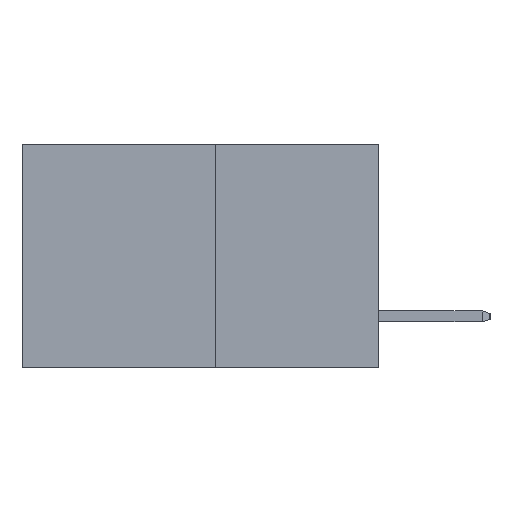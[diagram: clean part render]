
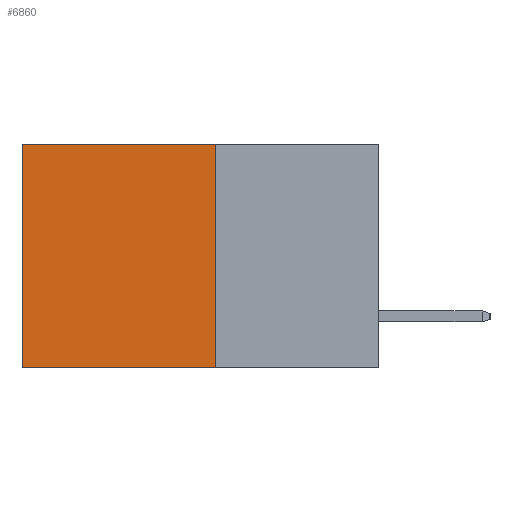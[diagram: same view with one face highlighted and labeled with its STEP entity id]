
A CAD part, left-side view. The second image highlights one B-rep face of the part: STEP entity #6860.
In plain terms, the highlighted planar face has unit normal (-1, 0, 0).
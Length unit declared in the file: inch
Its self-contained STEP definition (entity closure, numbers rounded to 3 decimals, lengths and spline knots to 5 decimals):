
#14 = PLANE ( 'NONE',  #4374 ) ;
#147 = LINE ( 'NONE', #5275, #4679 ) ;
#233 = LINE ( 'NONE', #394, #4769 ) ;
#394 = CARTESIAN_POINT ( 'NONE',  ( 0.277, 0.27, -0.37 ) ) ;
#927 = EDGE_CURVE ( 'NONE', #1650, #7988, #4878, .T. ) ;
#1343 = EDGE_CURVE ( 'NONE', #1881, #6970, #4865, .T. ) ;
#1384 = ORIENTED_EDGE ( 'NONE', *, *, #1343, .T. ) ;
#1650 = VERTEX_POINT ( 'NONE', #10716 ) ;
#1881 = VERTEX_POINT ( 'NONE', #8391 ) ;
#1893 = DIRECTION ( 'NONE',  ( 1., 0., 0. ) ) ;
#2575 = CARTESIAN_POINT ( 'NONE',  ( 0.277, 0.27, -0.37 ) ) ;
#3028 = FACE_OUTER_BOUND ( 'NONE', #7648, .T. ) ;
#3999 = ORIENTED_EDGE ( 'NONE', *, *, #5918, .F. ) ;
#4323 = VECTOR ( 'NONE', #5070, 39.37008 ) ;
#4374 = AXIS2_PLACEMENT_3D ( 'NONE', #7253, #1893, #8123 ) ;
#4579 = VECTOR ( 'NONE', #7801, 39.37008 ) ;
#4679 = VECTOR ( 'NONE', #6206, 39.37008 ) ;
#4769 = VECTOR ( 'NONE', #6738, 39.37008 ) ;
#4865 = LINE ( 'NONE', #9059, #4579 ) ;
#4878 = LINE ( 'NONE', #2575, #4323 ) ;
#5070 = DIRECTION ( 'NONE',  ( 0., 0., -1. ) ) ;
#5275 = CARTESIAN_POINT ( 'NONE',  ( 0.277, 0.27, 0. ) ) ;
#5918 = EDGE_CURVE ( 'NONE', #7988, #6970, #233, .T. ) ;
#6206 = DIRECTION ( 'NONE',  ( 0., 1., 0. ) ) ;
#6727 = EDGE_CURVE ( 'NONE', #1650, #1881, #147, .T. ) ;
#6738 = DIRECTION ( 'NONE',  ( 0., 1., 0. ) ) ;
#6757 = ORIENTED_EDGE ( 'NONE', *, *, #6727, .T. ) ;
#6860 = ADVANCED_FACE ( 'NONE', ( #3028 ), #14, .F. ) ;
#6970 = VERTEX_POINT ( 'NONE', #9967 ) ;
#7253 = CARTESIAN_POINT ( 'NONE',  ( 0.277, 0.27, -0.37 ) ) ;
#7648 = EDGE_LOOP ( 'NONE', ( #1384, #3999, #8847, #6757 ) ) ;
#7801 = DIRECTION ( 'NONE',  ( 0., 0., -1. ) ) ;
#7948 = CARTESIAN_POINT ( 'NONE',  ( 0.277, 0.27, -0.37 ) ) ;
#7988 = VERTEX_POINT ( 'NONE', #7948 ) ;
#8123 = DIRECTION ( 'NONE',  ( 0., 0., -1. ) ) ;
#8391 = CARTESIAN_POINT ( 'NONE',  ( 0.277, 0.59, 0. ) ) ;
#8847 = ORIENTED_EDGE ( 'NONE', *, *, #927, .F. ) ;
#9059 = CARTESIAN_POINT ( 'NONE',  ( 0.277, 0.59, -0.37 ) ) ;
#9967 = CARTESIAN_POINT ( 'NONE',  ( 0.277, 0.59, -0.37 ) ) ;
#10716 = CARTESIAN_POINT ( 'NONE',  ( 0.277, 0.27, 0. ) ) ;
